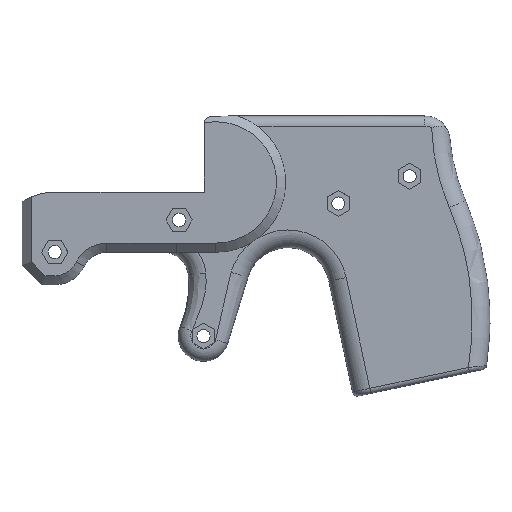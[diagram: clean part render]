
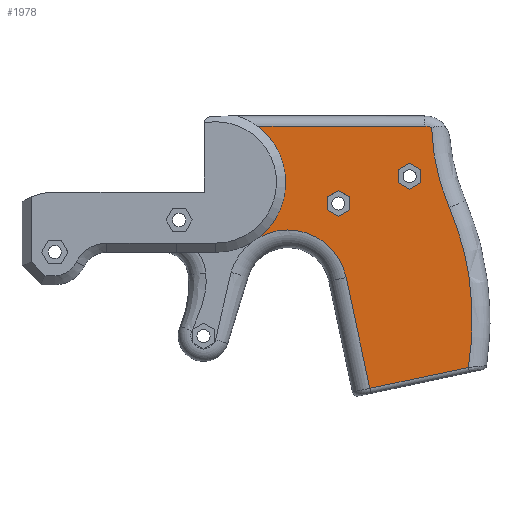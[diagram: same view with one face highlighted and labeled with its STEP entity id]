
A CAD part, top view. The second image highlights one B-rep face of the part: STEP entity #1978.
In plain terms, the highlighted planar face has unit normal (0, 0, 1).
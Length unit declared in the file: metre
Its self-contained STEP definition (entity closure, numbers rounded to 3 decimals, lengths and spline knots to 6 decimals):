
#93=CIRCLE('',#2108,0.071755);
#94=CIRCLE('',#2109,0.071755);
#95=CIRCLE('',#2110,0.055245);
#96=CIRCLE('',#2111,0.00381);
#97=CIRCLE('',#2112,0.017526);
#98=CIRCLE('',#2113,0.014949);
#158=ORIENTED_EDGE('',*,*,#748,.F.);
#159=ORIENTED_EDGE('',*,*,#749,.F.);
#160=ORIENTED_EDGE('',*,*,#750,.F.);
#161=ORIENTED_EDGE('',*,*,#751,.F.);
#162=ORIENTED_EDGE('',*,*,#752,.F.);
#163=ORIENTED_EDGE('',*,*,#753,.F.);
#164=ORIENTED_EDGE('',*,*,#754,.F.);
#165=ORIENTED_EDGE('',*,*,#755,.F.);
#166=ORIENTED_EDGE('',*,*,#756,.F.);
#167=ORIENTED_EDGE('',*,*,#757,.F.);
#168=ORIENTED_EDGE('',*,*,#758,.F.);
#169=ORIENTED_EDGE('',*,*,#759,.F.);
#170=ORIENTED_EDGE('',*,*,#760,.F.);
#171=ORIENTED_EDGE('',*,*,#761,.T.);
#172=ORIENTED_EDGE('',*,*,#762,.F.);
#173=ORIENTED_EDGE('',*,*,#763,.F.);
#174=ORIENTED_EDGE('',*,*,#764,.F.);
#175=ORIENTED_EDGE('',*,*,#765,.F.);
#176=ORIENTED_EDGE('',*,*,#766,.T.);
#177=ORIENTED_EDGE('',*,*,#767,.F.);
#178=ORIENTED_EDGE('',*,*,#768,.F.);
#179=ORIENTED_EDGE('',*,*,#769,.F.);
#748=EDGE_CURVE('',#1043,#1044,#1239,.T.);
#749=EDGE_CURVE('',#1045,#1043,#1240,.T.);
#750=EDGE_CURVE('',#1046,#1045,#1241,.T.);
#751=EDGE_CURVE('',#1047,#1046,#1242,.T.);
#752=EDGE_CURVE('',#1048,#1047,#1243,.T.);
#753=EDGE_CURVE('',#1044,#1048,#1244,.T.);
#754=EDGE_CURVE('',#1049,#1050,#1245,.T.);
#755=EDGE_CURVE('',#1051,#1049,#1246,.T.);
#756=EDGE_CURVE('',#1052,#1051,#1247,.T.);
#757=EDGE_CURVE('',#1053,#1052,#1248,.T.);
#758=EDGE_CURVE('',#1054,#1053,#1249,.T.);
#759=EDGE_CURVE('',#1050,#1054,#1250,.T.);
#760=EDGE_CURVE('',#1055,#1056,#93,.T.);
#761=EDGE_CURVE('',#1055,#1057,#1251,.T.);
#762=EDGE_CURVE('',#1058,#1057,#94,.T.);
#763=EDGE_CURVE('',#1059,#1058,#95,.F.);
#764=EDGE_CURVE('',#1060,#1059,#96,.T.);
#765=EDGE_CURVE('',#1061,#1060,#1252,.F.);
#766=EDGE_CURVE('',#1061,#1062,#97,.T.);
#767=EDGE_CURVE('',#1063,#1062,#98,.F.);
#768=EDGE_CURVE('',#1064,#1063,#1253,.T.);
#769=EDGE_CURVE('',#1056,#1064,#1254,.T.);
#1043=VERTEX_POINT('',#2850);
#1044=VERTEX_POINT('',#2851);
#1045=VERTEX_POINT('',#2853);
#1046=VERTEX_POINT('',#2855);
#1047=VERTEX_POINT('',#2857);
#1048=VERTEX_POINT('',#2859);
#1049=VERTEX_POINT('',#2862);
#1050=VERTEX_POINT('',#2863);
#1051=VERTEX_POINT('',#2865);
#1052=VERTEX_POINT('',#2867);
#1053=VERTEX_POINT('',#2869);
#1054=VERTEX_POINT('',#2871);
#1055=VERTEX_POINT('',#2874);
#1056=VERTEX_POINT('',#2875);
#1057=VERTEX_POINT('',#2877);
#1058=VERTEX_POINT('',#2879);
#1059=VERTEX_POINT('',#2881);
#1060=VERTEX_POINT('',#2883);
#1061=VERTEX_POINT('',#2885);
#1062=VERTEX_POINT('',#2887);
#1063=VERTEX_POINT('',#2889);
#1064=VERTEX_POINT('',#2891);
#1239=LINE('',#2849,#1431);
#1240=LINE('',#2852,#1432);
#1241=LINE('',#2854,#1433);
#1242=LINE('',#2856,#1434);
#1243=LINE('',#2858,#1435);
#1244=LINE('',#2860,#1436);
#1245=LINE('',#2861,#1437);
#1246=LINE('',#2864,#1438);
#1247=LINE('',#2866,#1439);
#1248=LINE('',#2868,#1440);
#1249=LINE('',#2870,#1441);
#1250=LINE('',#2872,#1442);
#1251=LINE('',#2876,#1443);
#1252=LINE('',#2884,#1444);
#1253=LINE('',#2890,#1445);
#1254=LINE('',#2892,#1446);
#1431=VECTOR('',#2293,1.);
#1432=VECTOR('',#2294,1.);
#1433=VECTOR('',#2295,1.);
#1434=VECTOR('',#2296,1.);
#1435=VECTOR('',#2297,1.);
#1436=VECTOR('',#2298,1.);
#1437=VECTOR('',#2299,1.);
#1438=VECTOR('',#2300,1.);
#1439=VECTOR('',#2301,1.);
#1440=VECTOR('',#2302,1.);
#1441=VECTOR('',#2303,1.);
#1442=VECTOR('',#2304,1.);
#1443=VECTOR('',#2307,1.);
#1444=VECTOR('',#2314,1.);
#1445=VECTOR('',#2319,1.);
#1446=VECTOR('',#2320,1.);
#1623=EDGE_LOOP('',(#158,#159,#160,#161,#162,#163));
#1624=EDGE_LOOP('',(#164,#165,#166,#167,#168,#169));
#1625=EDGE_LOOP('',(#170,#171,#172,#173,#174,#175,#176,#177,#178,#179));
#1764=FACE_BOUND('',#1623,.T.);
#1765=FACE_BOUND('',#1624,.T.);
#1766=FACE_BOUND('',#1625,.T.);
#1905=PLANE('',#2107);
#1978=ADVANCED_FACE('',(#1764,#1765,#1766),#1905,.T.);
#2107=AXIS2_PLACEMENT_3D('',#2848,#2291,#2292);
#2108=AXIS2_PLACEMENT_3D('',#2873,#2305,#2306);
#2109=AXIS2_PLACEMENT_3D('',#2878,#2308,#2309);
#2110=AXIS2_PLACEMENT_3D('',#2880,#2310,#2311);
#2111=AXIS2_PLACEMENT_3D('',#2882,#2312,#2313);
#2112=AXIS2_PLACEMENT_3D('',#2886,#2315,#2316);
#2113=AXIS2_PLACEMENT_3D('',#2888,#2317,#2318);
#2291=DIRECTION('',(0.,0.,1.));
#2292=DIRECTION('',(-1.,0.,0.));
#2293=DIRECTION('',(-0.866,-0.5,0.));
#2294=DIRECTION('',(-0.866,0.5,0.));
#2295=DIRECTION('',(0.,1.,0.));
#2296=DIRECTION('',(0.866,0.5,0.));
#2297=DIRECTION('',(0.866,-0.5,0.));
#2298=DIRECTION('',(0.,-1.,0.));
#2299=DIRECTION('',(0.866,0.5,0.));
#2300=DIRECTION('',(0.866,-0.5,0.));
#2301=DIRECTION('',(0.,-1.,0.));
#2302=DIRECTION('',(-0.866,-0.5,0.));
#2303=DIRECTION('',(-0.866,0.5,0.));
#2304=DIRECTION('',(0.,1.,0.));
#2305=DIRECTION('',(0.,0.,-1.));
#2306=DIRECTION('',(-1.,0.,0.));
#2307=DIRECTION('',(-0.131,0.991,0.));
#2308=DIRECTION('',(0.,0.,-1.));
#2309=DIRECTION('',(-1.,0.,0.));
#2310=DIRECTION('',(0.,0.,-1.));
#2311=DIRECTION('',(-1.,0.,0.));
#2312=DIRECTION('',(0.,0.,-1.));
#2313=DIRECTION('',(-1.,0.,0.));
#2314=DIRECTION('',(-1.,0.,0.));
#2315=DIRECTION('',(0.,0.,-1.));
#2316=DIRECTION('',(-1.,0.,0.));
#2317=DIRECTION('',(0.,0.,-1.));
#2318=DIRECTION('',(-1.,0.,0.));
#2319=DIRECTION('',(-0.208,0.978,0.));
#2320=DIRECTION('',(-0.978,-0.208,0.));
#2848=CARTESIAN_POINT('',(0.102328,0.021885,-0.017426));
#2849=CARTESIAN_POINT('',(0.143043,0.038903,-0.017426));
#2850=CARTESIAN_POINT('',(0.144459,0.03972,-0.017426));
#2851=CARTESIAN_POINT('',(0.141627,0.038085,-0.017426));
#2852=CARTESIAN_POINT('',(0.145875,0.038903,-0.017426));
#2853=CARTESIAN_POINT('',(0.147291,0.038085,-0.017426));
#2854=CARTESIAN_POINT('',(0.147291,0.03645,-0.017426));
#2855=CARTESIAN_POINT('',(0.147291,0.034815,-0.017426));
#2856=CARTESIAN_POINT('',(0.145875,0.033997,-0.017426));
#2857=CARTESIAN_POINT('',(0.144459,0.03318,-0.017426));
#2858=CARTESIAN_POINT('',(0.143043,0.033997,-0.017426));
#2859=CARTESIAN_POINT('',(0.141627,0.034815,-0.017426));
#2860=CARTESIAN_POINT('',(0.141627,0.03645,-0.017426));
#2861=CARTESIAN_POINT('',(0.106457,0.014735,-0.017426));
#2862=CARTESIAN_POINT('',(0.126558,0.02634,-0.017426));
#2863=CARTESIAN_POINT('',(0.12939,0.027975,-0.017426));
#2864=CARTESIAN_POINT('',(0.110315,0.035718,-0.017426));
#2865=CARTESIAN_POINT('',(0.123726,0.027975,-0.017426));
#2866=CARTESIAN_POINT('',(0.123726,0.021885,-0.017426));
#2867=CARTESIAN_POINT('',(0.123726,0.031245,-0.017426));
#2868=CARTESIAN_POINT('',(0.103625,0.01964,-0.017426));
#2869=CARTESIAN_POINT('',(0.126558,0.032881,-0.017426));
#2870=CARTESIAN_POINT('',(0.113147,0.040623,-0.017426));
#2871=CARTESIAN_POINT('',(0.12939,0.031245,-0.017426));
#2872=CARTESIAN_POINT('',(0.12939,0.021885,-0.017426));
#2873=CARTESIAN_POINT('',(0.088447,0.00034,-0.017426));
#2874=CARTESIAN_POINT('',(0.159349,0.011363,-0.017426));
#2875=CARTESIAN_POINT('',(0.15921,-0.011553,-0.017426));
#2876=CARTESIAN_POINT('',(0.159563,0.009744,-0.017426));
#2877=CARTESIAN_POINT('',(0.159338,0.01144,-0.017426));
#2878=CARTESIAN_POINT('',(0.088447,0.00034,-0.017426));
#2879=CARTESIAN_POINT('',(0.154411,0.028581,-0.017426));
#2880=CARTESIAN_POINT('',(0.205197,0.050324,-0.017426));
#2881=CARTESIAN_POINT('',(0.149978,0.048651,-0.017426));
#2882=CARTESIAN_POINT('',(0.148274,0.045244,-0.017426));
#2883=CARTESIAN_POINT('',(0.148274,0.049054,-0.017426));
#2884=CARTESIAN_POINT('',(0.148274,0.049054,-0.017426));
#2885=CARTESIAN_POINT('',(0.10613,0.049054,-0.017426));
#2886=CARTESIAN_POINT('',(0.095806,0.034891,-0.017426));
#2887=CARTESIAN_POINT('',(0.106372,0.020909,-0.017426));
#2888=CARTESIAN_POINT('',(0.11392,0.008005,-0.017426));
#2889=CARTESIAN_POINT('',(0.128559,0.011035,-0.017426));
#2890=CARTESIAN_POINT('',(0.128553,0.01106,-0.017426));
#2891=CARTESIAN_POINT('',(0.134477,-0.01681,-0.017426));
#2892=CARTESIAN_POINT('',(0.134477,-0.01681,-0.017426));
